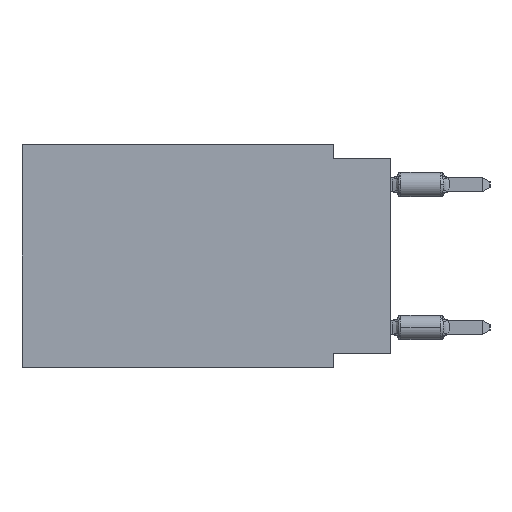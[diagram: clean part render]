
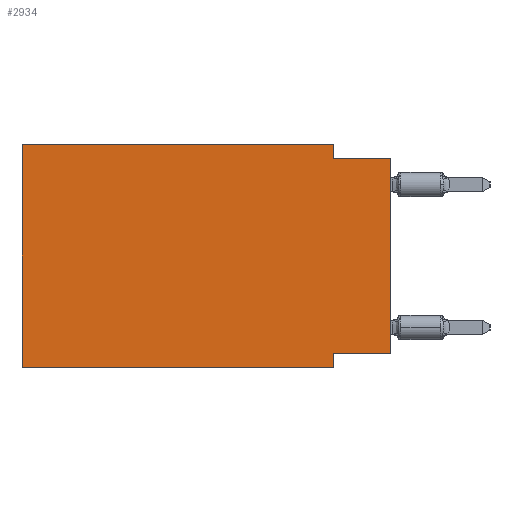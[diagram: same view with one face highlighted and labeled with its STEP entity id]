
A CAD part, left-side view. The second image highlights one B-rep face of the part: STEP entity #2934.
In plain terms, the highlighted planar face has unit normal (-1, 0, 0).
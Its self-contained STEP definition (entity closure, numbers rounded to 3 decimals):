
#615 = VECTOR ( 'NONE', #33393, 1000. ) ;
#2110 = VERTEX_POINT ( 'NONE', #21984 ) ;
#2376 = AXIS2_PLACEMENT_3D ( 'NONE', #11215, #26108, #31941 ) ;
#2396 = CARTESIAN_POINT ( 'NONE',  ( 0., 16.383, 0. ) ) ;
#2435 = VERTEX_POINT ( 'NONE', #34633 ) ;
#2934 = ADVANCED_FACE ( 'NONE', ( #38196 ), #17447, .F. ) ;
#4371 = ORIENTED_EDGE ( 'NONE', *, *, #15287, .T. ) ;
#5032 = EDGE_CURVE ( 'NONE', #39240, #33160, #13156, .T. ) ;
#5879 = EDGE_CURVE ( 'NONE', #2435, #34998, #24548, .T. ) ;
#7161 = CARTESIAN_POINT ( 'NONE',  ( 0., 2.54, -0.635 ) ) ;
#7398 = DIRECTION ( 'NONE',  ( 0., 0., -1. ) ) ;
#7860 = LINE ( 'NONE', #20129, #27460 ) ;
#8497 = EDGE_CURVE ( 'NONE', #2110, #24358, #32225, .T. ) ;
#10420 = CARTESIAN_POINT ( 'NONE',  ( 0., 2.54, 0. ) ) ;
#10495 = CARTESIAN_POINT ( 'NONE',  ( 0., 2.54, -9.906 ) ) ;
#11215 = CARTESIAN_POINT ( 'NONE',  ( 0., 16.383, 0. ) ) ;
#11985 = EDGE_CURVE ( 'NONE', #2110, #39240, #34362, .T. ) ;
#13156 = LINE ( 'NONE', #28270, #17921 ) ;
#13518 = CARTESIAN_POINT ( 'NONE',  ( 0., 0., 0. ) ) ;
#14294 = DIRECTION ( 'NONE',  ( 0., -1., 0. ) ) ;
#15287 = EDGE_CURVE ( 'NONE', #2435, #33160, #30574, .T. ) ;
#15677 = DIRECTION ( 'NONE',  ( 0., 0., 1. ) ) ;
#16037 = DIRECTION ( 'NONE',  ( 0., 1., 0. ) ) ;
#16156 = VERTEX_POINT ( 'NONE', #7161 ) ;
#16531 = DIRECTION ( 'NONE',  ( 0., 0., 1. ) ) ;
#16943 = VECTOR ( 'NONE', #32996, 1000. ) ;
#17447 = PLANE ( 'NONE',  #2376 ) ;
#17921 = VECTOR ( 'NONE', #28649, 1000. ) ;
#18508 = CARTESIAN_POINT ( 'NONE',  ( 0., 16.383, 0. ) ) ;
#18678 = EDGE_CURVE ( 'NONE', #33381, #16156, #20263, .T. ) ;
#19059 = CARTESIAN_POINT ( 'NONE',  ( 0., 0., -9.271 ) ) ;
#19839 = CARTESIAN_POINT ( 'NONE',  ( 0., 2.54, -9.271 ) ) ;
#19929 = ORIENTED_EDGE ( 'NONE', *, *, #8497, .T. ) ;
#19972 = ORIENTED_EDGE ( 'NONE', *, *, #27273, .F. ) ;
#20129 = CARTESIAN_POINT ( 'NONE',  ( 0., 0., -0.635 ) ) ;
#20263 = LINE ( 'NONE', #10420, #24549 ) ;
#21984 = CARTESIAN_POINT ( 'NONE',  ( 0., 0., -9.271 ) ) ;
#22629 = VECTOR ( 'NONE', #16531, 1000. ) ;
#23062 = ORIENTED_EDGE ( 'NONE', *, *, #18678, .F. ) ;
#23541 = LINE ( 'NONE', #35833, #16943 ) ;
#24358 = VERTEX_POINT ( 'NONE', #37258 ) ;
#24548 = LINE ( 'NONE', #18508, #34715 ) ;
#24549 = VECTOR ( 'NONE', #7398, 1000. ) ;
#26108 = DIRECTION ( 'NONE',  ( 1., 0., 0. ) ) ;
#26818 = VECTOR ( 'NONE', #16037, 1000. ) ;
#27273 = EDGE_CURVE ( 'NONE', #16156, #24358, #7860, .T. ) ;
#27460 = VECTOR ( 'NONE', #14294, 1000. ) ;
#28270 = CARTESIAN_POINT ( 'NONE',  ( 0., 2.54, -9.906 ) ) ;
#28452 = ORIENTED_EDGE ( 'NONE', *, *, #37346, .F. ) ;
#28511 = ORIENTED_EDGE ( 'NONE', *, *, #11985, .F. ) ;
#28649 = DIRECTION ( 'NONE',  ( 0., 0., -1. ) ) ;
#29021 = ORIENTED_EDGE ( 'NONE', *, *, #5879, .F. ) ;
#29755 = EDGE_LOOP ( 'NONE', ( #19929, #19972, #23062, #28452, #29021, #4371, #37684, #28511 ) ) ;
#30574 = LINE ( 'NONE', #33793, #615 ) ;
#31941 = DIRECTION ( 'NONE',  ( 0., 0., -1. ) ) ;
#32225 = LINE ( 'NONE', #13518, #22629 ) ;
#32996 = DIRECTION ( 'NONE',  ( 0., -1., 0. ) ) ;
#33160 = VERTEX_POINT ( 'NONE', #10495 ) ;
#33381 = VERTEX_POINT ( 'NONE', #36051 ) ;
#33393 = DIRECTION ( 'NONE',  ( 0., -1., 0. ) ) ;
#33793 = CARTESIAN_POINT ( 'NONE',  ( 0., 16.383, -9.906 ) ) ;
#34362 = LINE ( 'NONE', #19059, #26818 ) ;
#34633 = CARTESIAN_POINT ( 'NONE',  ( 0., 16.383, -9.906 ) ) ;
#34715 = VECTOR ( 'NONE', #15677, 1000. ) ;
#34998 = VERTEX_POINT ( 'NONE', #2396 ) ;
#35833 = CARTESIAN_POINT ( 'NONE',  ( 0., 16.383, 0. ) ) ;
#36051 = CARTESIAN_POINT ( 'NONE',  ( 0., 2.54, 0. ) ) ;
#37258 = CARTESIAN_POINT ( 'NONE',  ( 0., 0., -0.635 ) ) ;
#37346 = EDGE_CURVE ( 'NONE', #34998, #33381, #23541, .T. ) ;
#37684 = ORIENTED_EDGE ( 'NONE', *, *, #5032, .F. ) ;
#38196 = FACE_OUTER_BOUND ( 'NONE', #29755, .T. ) ;
#39240 = VERTEX_POINT ( 'NONE', #19839 ) ;
